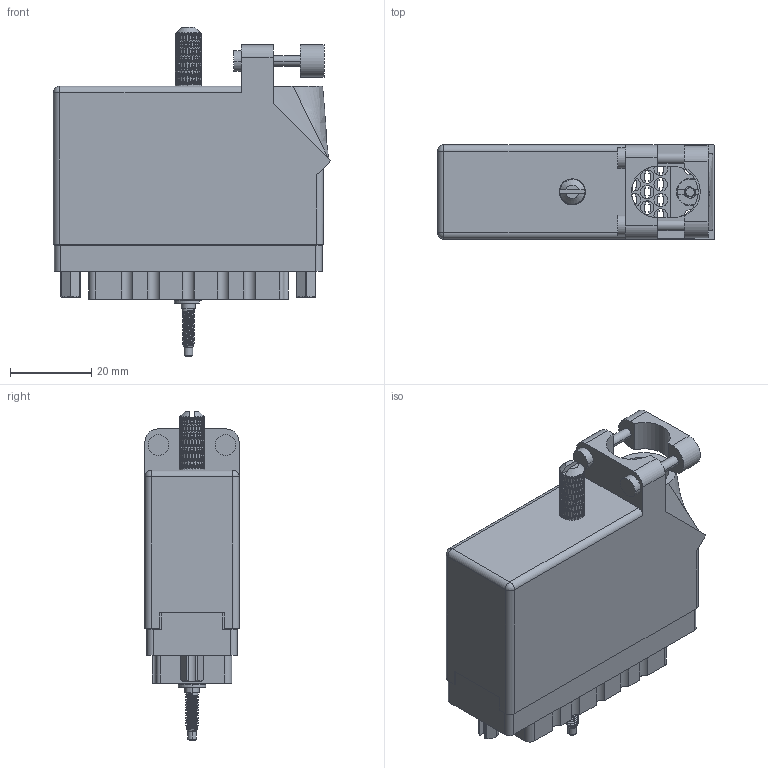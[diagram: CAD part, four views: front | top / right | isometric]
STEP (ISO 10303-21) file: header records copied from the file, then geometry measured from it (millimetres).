
FILE_DESCRIPTION (( 'STEP AP203' ), '1' );
FILE_NAME ('516-056-000-411.STEP', '2020-03-05T19:57:44', ( '' ), ( '' ), 'SwSTEP 2.0', 'SolidWorks 2016', '' );
FILE_SCHEMA (( 'CONFIG_CONTROL_DESIGN' ));
Length unit declared in the file: inch
Products named in the file (11): 516-221-038-102_057; 516 Part Receptacle_056; 516-251-035-100; 516-253-035-100; 516-250-038-111; 516-253-138-107; Actuating Screw Assy 038-056; 516-252-021-102_056; 516-230-001_Plastic - 056 Top Entry; 516-221-038-102_056; 516-056-000-411
Assembly tree (12 placements, depth 3):
  516-056-000-411
    516 Part Receptacle_056
    516-230-001_Plastic - 056 Top Entry
    516-252-021-102_056  x2
    516-221-038-102_056
    Actuating Screw Assy 038-056
      516-251-035-100
      516-253-035-100  x2
      516-253-138-107
      516-250-038-111
    516-221-038-102_057
Bounding box: 68.14 x 23.11 x 81.03 mm (x, y, z)
Volume: 29014.7 mm3; surface area: 39823.5 mm2
Topology: 11 solids, 11 shells, 2904 faces, 7382 edges, 4520 vertices
Faces by surface type: plane 1053, bspline 1037, cylinder 760, cone 52, sphere 2
Entity records: 120527 total; most frequent: CARTESIAN_POINT 61415, ORIENTED_EDGE 14548, DIRECTION 9450, EDGE_CURVE 7274, VERTEX_POINT 4452, AXIS2_PLACEMENT_3D 3165, LINE 3120, VECTOR 3120
